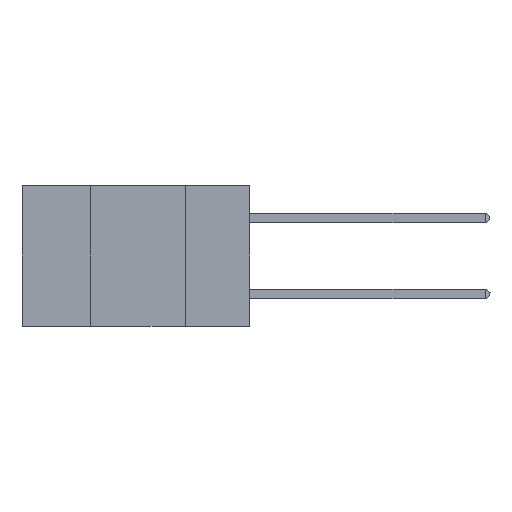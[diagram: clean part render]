
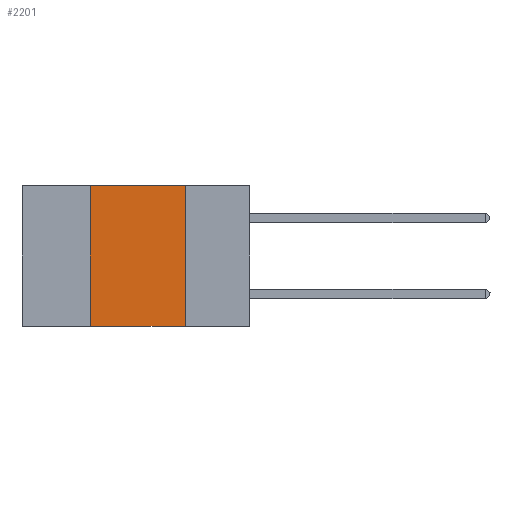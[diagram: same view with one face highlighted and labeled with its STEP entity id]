
A CAD part, left-side view. The second image highlights one B-rep face of the part: STEP entity #2201.
In plain terms, the highlighted planar face has unit normal (-1, 0, 0).
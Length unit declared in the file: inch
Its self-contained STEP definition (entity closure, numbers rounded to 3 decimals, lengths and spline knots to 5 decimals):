
#78 = VECTOR ( 'NONE', #6941, 39.37008 ) ;
#159 = VECTOR ( 'NONE', #9913, 39.37008 ) ;
#701 = ORIENTED_EDGE ( 'NONE', *, *, #5307, .F. ) ;
#1450 = LINE ( 'NONE', #10696, #8411 ) ;
#1699 = CARTESIAN_POINT ( 'NONE',  ( 0., 0.17, 0. ) ) ;
#2201 = ADVANCED_FACE ( 'NONE', ( #14413 ), #9687, .F. ) ;
#2480 = VERTEX_POINT ( 'NONE', #14640 ) ;
#3978 = VERTEX_POINT ( 'NONE', #8289 ) ;
#4371 = CARTESIAN_POINT ( 'NONE',  ( 0., 0.6, -0.37 ) ) ;
#4592 = AXIS2_PLACEMENT_3D ( 'NONE', #16554, #8345, #5412 ) ;
#4707 = DIRECTION ( 'NONE',  ( 0., 0., 1. ) ) ;
#4983 = EDGE_CURVE ( 'NONE', #3978, #11714, #14771, .T. ) ;
#5307 = EDGE_CURVE ( 'NONE', #2480, #3978, #1450, .T. ) ;
#5335 = LINE ( 'NONE', #4371, #78 ) ;
#5412 = DIRECTION ( 'NONE',  ( 0., 0., -1. ) ) ;
#6933 = EDGE_CURVE ( 'NONE', #12482, #11714, #5335, .T. ) ;
#6941 = DIRECTION ( 'NONE',  ( 0., -1., 0. ) ) ;
#8172 = VECTOR ( 'NONE', #4707, 39.37008 ) ;
#8289 = CARTESIAN_POINT ( 'NONE',  ( 0., 0.17, 0. ) ) ;
#8345 = DIRECTION ( 'NONE',  ( 1., 0., 0. ) ) ;
#8411 = VECTOR ( 'NONE', #16405, 39.37008 ) ;
#8472 = ORIENTED_EDGE ( 'NONE', *, *, #6933, .T. ) ;
#9687 = PLANE ( 'NONE',  #4592 ) ;
#9913 = DIRECTION ( 'NONE',  ( 0., 0., -1. ) ) ;
#10642 = ORIENTED_EDGE ( 'NONE', *, *, #16898, .F. ) ;
#10696 = CARTESIAN_POINT ( 'NONE',  ( 0., 0.6, 0. ) ) ;
#11647 = LINE ( 'NONE', #17142, #8172 ) ;
#11714 = VERTEX_POINT ( 'NONE', #13144 ) ;
#12482 = VERTEX_POINT ( 'NONE', #17329 ) ;
#13144 = CARTESIAN_POINT ( 'NONE',  ( 0., 0.17, -0.37 ) ) ;
#14413 = FACE_OUTER_BOUND ( 'NONE', #15528, .T. ) ;
#14640 = CARTESIAN_POINT ( 'NONE',  ( 0., 0.42, 0. ) ) ;
#14771 = LINE ( 'NONE', #1699, #159 ) ;
#15528 = EDGE_LOOP ( 'NONE', ( #16615, #701, #10642, #8472 ) ) ;
#16405 = DIRECTION ( 'NONE',  ( 0., -1., 0. ) ) ;
#16554 = CARTESIAN_POINT ( 'NONE',  ( 0., 0.6, 0. ) ) ;
#16615 = ORIENTED_EDGE ( 'NONE', *, *, #4983, .F. ) ;
#16898 = EDGE_CURVE ( 'NONE', #12482, #2480, #11647, .T. ) ;
#17142 = CARTESIAN_POINT ( 'NONE',  ( 0., 0.42, 0. ) ) ;
#17329 = CARTESIAN_POINT ( 'NONE',  ( 0., 0.42, -0.37 ) ) ;
